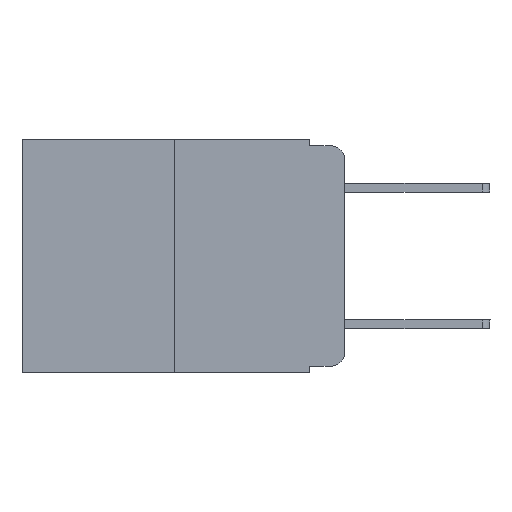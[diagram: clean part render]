
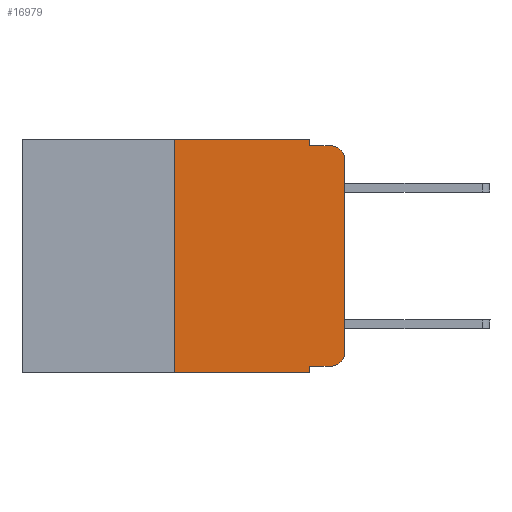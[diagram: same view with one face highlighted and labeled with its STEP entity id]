
A CAD part, left-side view. The second image highlights one B-rep face of the part: STEP entity #16979.
In plain terms, the highlighted planar face has unit normal (-1, 0, 0).
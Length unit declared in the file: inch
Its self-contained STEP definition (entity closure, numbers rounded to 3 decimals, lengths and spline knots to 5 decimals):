
#394 = VERTEX_POINT ( 'NONE', #15309 ) ;
#507 = LINE ( 'NONE', #8946, #11630 ) ;
#604 = VERTEX_POINT ( 'NONE', #1266 ) ;
#921 = CARTESIAN_POINT ( 'NONE',  ( 0., 0.02, -0.01 ) ) ;
#1120 = CARTESIAN_POINT ( 'NONE',  ( 0., 0.25, 0. ) ) ;
#1266 = CARTESIAN_POINT ( 'NONE',  ( 0., 0.25, -0.343 ) ) ;
#1589 = VECTOR ( 'NONE', #14294, 39.37008 ) ;
#1607 = EDGE_CURVE ( 'NONE', #394, #2727, #5610, .T. ) ;
#2046 = EDGE_CURVE ( 'NONE', #2727, #6802, #6334, .T. ) ;
#2218 = ORIENTED_EDGE ( 'NONE', *, *, #7444, .F. ) ;
#2389 = LINE ( 'NONE', #13656, #10227 ) ;
#2411 = DIRECTION ( 'NONE',  ( 0., -1., 0. ) ) ;
#2700 = CARTESIAN_POINT ( 'NONE',  ( 0., 0.473, 0. ) ) ;
#2727 = VERTEX_POINT ( 'NONE', #3275 ) ;
#2831 = EDGE_CURVE ( 'NONE', #604, #6323, #9792, .T. ) ;
#2970 = EDGE_LOOP ( 'NONE', ( #9641, #7909, #2218, #7148, #3705, #10270, #15044, #11222, #11092, #11831 ) ) ;
#3115 = CARTESIAN_POINT ( 'NONE',  ( 0., 0.051, 0. ) ) ;
#3275 = CARTESIAN_POINT ( 'NONE',  ( 0., 0., -0.03 ) ) ;
#3475 = CARTESIAN_POINT ( 'NONE',  ( 0., 0., 0. ) ) ;
#3705 = ORIENTED_EDGE ( 'NONE', *, *, #7343, .F. ) ;
#4081 = AXIS2_PLACEMENT_3D ( 'NONE', #2700, #6665, #11920 ) ;
#4316 = DIRECTION ( 'NONE',  ( 0., -1., 0. ) ) ;
#4401 = DIRECTION ( 'NONE',  ( 0., 0., 1. ) ) ;
#4905 = DIRECTION ( 'NONE',  ( 0., -1., 0. ) ) ;
#4963 = CARTESIAN_POINT ( 'NONE',  ( 0., 0.473, 0. ) ) ;
#5025 = DIRECTION ( 'NONE',  ( 0., 0., -1. ) ) ;
#5113 = VERTEX_POINT ( 'NONE', #11941 ) ;
#5175 = VERTEX_POINT ( 'NONE', #7979 ) ;
#5215 = VECTOR ( 'NONE', #8803, 39.37008 ) ;
#5610 = LINE ( 'NONE', #3475, #5215 ) ;
#5623 = EDGE_CURVE ( 'NONE', #11232, #6062, #8462, .T. ) ;
#6062 = VERTEX_POINT ( 'NONE', #13513 ) ;
#6121 = DIRECTION ( 'NONE',  ( 0., 0., -1. ) ) ;
#6323 = VERTEX_POINT ( 'NONE', #9015 ) ;
#6334 = CIRCLE ( 'NONE', #9384, 0.02 ) ;
#6397 = VECTOR ( 'NONE', #2411, 39.37008 ) ;
#6487 = VECTOR ( 'NONE', #4316, 39.37008 ) ;
#6665 = DIRECTION ( 'NONE',  ( 1., 0., 0. ) ) ;
#6802 = VERTEX_POINT ( 'NONE', #921 ) ;
#7079 = DIRECTION ( 'NONE',  ( 0., 0., -1. ) ) ;
#7148 = ORIENTED_EDGE ( 'NONE', *, *, #15014, .F. ) ;
#7335 = LINE ( 'NONE', #11656, #1589 ) ;
#7343 = EDGE_CURVE ( 'NONE', #14437, #5113, #16654, .T. ) ;
#7444 = EDGE_CURVE ( 'NONE', #5175, #6802, #7335, .T. ) ;
#7909 = ORIENTED_EDGE ( 'NONE', *, *, #2046, .T. ) ;
#7979 = CARTESIAN_POINT ( 'NONE',  ( 0., 0.051, -0.01 ) ) ;
#8462 = LINE ( 'NONE', #16952, #6397 ) ;
#8745 = DIRECTION ( 'NONE',  ( 0., 0., -1. ) ) ;
#8803 = DIRECTION ( 'NONE',  ( 0., 0., 1. ) ) ;
#8946 = CARTESIAN_POINT ( 'NONE',  ( 0., 0.051, 0. ) ) ;
#9015 = CARTESIAN_POINT ( 'NONE',  ( 0., 0.051, -0.343 ) ) ;
#9305 = CARTESIAN_POINT ( 'NONE',  ( 0., 0.051, -0.333 ) ) ;
#9384 = AXIS2_PLACEMENT_3D ( 'NONE', #14007, #15104, #8745 ) ;
#9641 = ORIENTED_EDGE ( 'NONE', *, *, #1607, .T. ) ;
#9792 = LINE ( 'NONE', #10804, #6487 ) ;
#10036 = VECTOR ( 'NONE', #4905, 39.37008 ) ;
#10227 = VECTOR ( 'NONE', #4401, 39.37008 ) ;
#10270 = ORIENTED_EDGE ( 'NONE', *, *, #13803, .F. ) ;
#10473 = VECTOR ( 'NONE', #7079, 39.37008 ) ;
#10804 = CARTESIAN_POINT ( 'NONE',  ( 0., 0.473, -0.343 ) ) ;
#11092 = ORIENTED_EDGE ( 'NONE', *, *, #5623, .T. ) ;
#11222 = ORIENTED_EDGE ( 'NONE', *, *, #11399, .F. ) ;
#11232 = VERTEX_POINT ( 'NONE', #9305 ) ;
#11399 = EDGE_CURVE ( 'NONE', #11232, #6323, #12120, .T. ) ;
#11630 = VECTOR ( 'NONE', #5025, 39.37008 ) ;
#11656 = CARTESIAN_POINT ( 'NONE',  ( 0., 0.051, -0.01 ) ) ;
#11831 = ORIENTED_EDGE ( 'NONE', *, *, #12300, .T. ) ;
#11920 = DIRECTION ( 'NONE',  ( 0., 0., -1. ) ) ;
#11941 = CARTESIAN_POINT ( 'NONE',  ( 0., 0.051, 0. ) ) ;
#12120 = LINE ( 'NONE', #3115, #10473 ) ;
#12300 = EDGE_CURVE ( 'NONE', #6062, #394, #14365, .T. ) ;
#12569 = CARTESIAN_POINT ( 'NONE',  ( 0., 0.02, -0.313 ) ) ;
#12620 = DIRECTION ( 'NONE',  ( -1., 0., 0. ) ) ;
#13513 = CARTESIAN_POINT ( 'NONE',  ( 0., 0.02, -0.333 ) ) ;
#13656 = CARTESIAN_POINT ( 'NONE',  ( 0., 0.25, 0. ) ) ;
#13776 = AXIS2_PLACEMENT_3D ( 'NONE', #12569, #12620, #6121 ) ;
#13803 = EDGE_CURVE ( 'NONE', #604, #14437, #2389, .T. ) ;
#14007 = CARTESIAN_POINT ( 'NONE',  ( 0., 0.02, -0.03 ) ) ;
#14294 = DIRECTION ( 'NONE',  ( 0., -1., 0. ) ) ;
#14365 = CIRCLE ( 'NONE', #13776, 0.02 ) ;
#14437 = VERTEX_POINT ( 'NONE', #1120 ) ;
#14865 = FACE_OUTER_BOUND ( 'NONE', #2970, .T. ) ;
#15014 = EDGE_CURVE ( 'NONE', #5113, #5175, #507, .T. ) ;
#15044 = ORIENTED_EDGE ( 'NONE', *, *, #2831, .T. ) ;
#15104 = DIRECTION ( 'NONE',  ( -1., 0., 0. ) ) ;
#15309 = CARTESIAN_POINT ( 'NONE',  ( 0., 0., -0.313 ) ) ;
#15908 = PLANE ( 'NONE',  #4081 ) ;
#16654 = LINE ( 'NONE', #4963, #10036 ) ;
#16952 = CARTESIAN_POINT ( 'NONE',  ( 0., 0.051, -0.333 ) ) ;
#16979 = ADVANCED_FACE ( 'NONE', ( #14865 ), #15908, .F. ) ;
